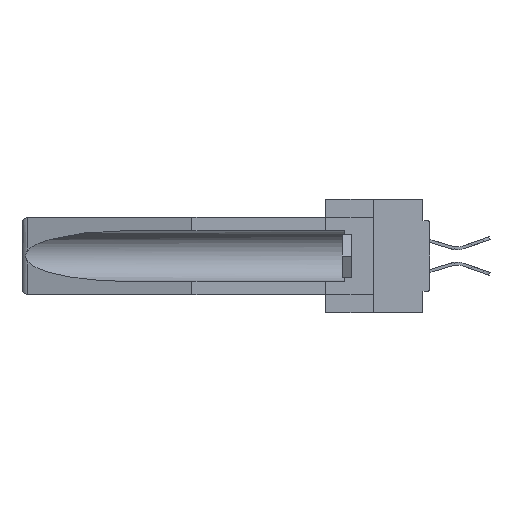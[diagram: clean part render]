
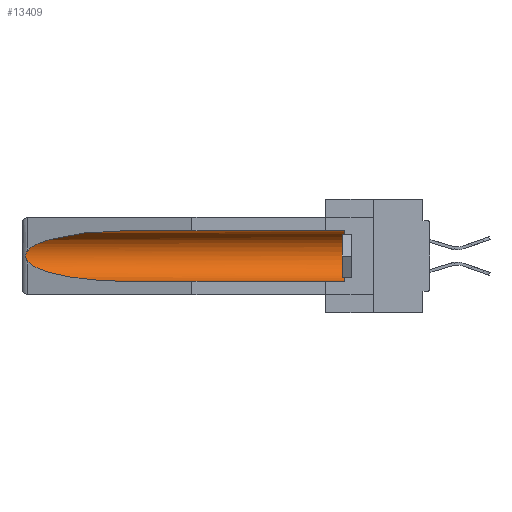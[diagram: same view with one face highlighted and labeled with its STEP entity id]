
A CAD part, left-side view. The second image highlights one B-rep face of the part: STEP entity #13409.
In plain terms, the highlighted cylindrical face has radius 2.857 mm (diameter 5.715 mm), a partial arc.
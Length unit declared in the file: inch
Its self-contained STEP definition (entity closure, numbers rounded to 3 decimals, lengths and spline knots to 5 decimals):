
#12 = AXIS2_PLACEMENT_3D ( 'NONE', #11659, #34735, #1858 ) ;
#1206 = CARTESIAN_POINT ( 'NONE',  ( 0.2675, 1.53308, -0.16763 ) ) ;
#1270 = DIRECTION ( 'NONE',  ( 0., 1., 0. ) ) ;
#1858 = DIRECTION ( 'NONE',  ( 0., 0., 1. ) ) ;
#2294 = CYLINDRICAL_SURFACE ( 'NONE', #33817, 0.1125 ) ;
#2442 = EDGE_CURVE ( 'NONE', #13617, #41362, #18137, .T. ) ;
#2776 = FACE_OUTER_BOUND ( 'NONE', #39328, .T. ) ;
#3018 = DIRECTION ( 'NONE',  ( 0., 1., 0. ) ) ;
#3958 = ORIENTED_EDGE ( 'NONE', *, *, #25917, .F. ) ;
#4309 = VECTOR ( 'NONE', #3018, 39.37008 ) ;
#4374 = CARTESIAN_POINT ( 'NONE',  ( 0.26654, 1.53092, -0.15636 ) ) ;
#5000 = CARTESIAN_POINT ( 'NONE',  ( 0.155, 1.07973, -0.284 ) ) ;
#5663 = CARTESIAN_POINT ( 'NONE',  ( 0.155, 0.126, -0.059 ) ) ;
#7551 = DIRECTION ( 'NONE',  ( 0., 0., 1. ) ) ;
#8029 = CARTESIAN_POINT ( 'NONE',  ( 0.21114, 1.30732, -0.284 ) ) ;
#8088 = EDGE_CURVE ( 'NONE', #12932, #9322, #22255, .T. ) ;
#8124 = EDGE_CURVE ( 'NONE', #18092, #32722, #23951, .T. ) ;
#9322 = VERTEX_POINT ( 'NONE', #5663 ) ;
#9747 = CARTESIAN_POINT ( 'NONE',  ( 0.155, -0.30754, -0.059 ) ) ;
#10079 = ORIENTED_EDGE ( 'NONE', *, *, #8088, .T. ) ;
#11659 = CARTESIAN_POINT ( 'NONE',  ( 0.155, 0.126, -0.1715 ) ) ;
#12932 = VERTEX_POINT ( 'NONE', #41295 ) ;
#13409 = ADVANCED_FACE ( 'NONE', ( #2776 ), #2294, .F. ) ;
#13617 = VERTEX_POINT ( 'NONE', #39685 ) ;
#14537 = CARTESIAN_POINT ( 'NONE',  ( 0.26537, 1.52718, -0.19328 ) ) ;
#15004 = ORIENTED_EDGE ( 'NONE', *, *, #2442, .T. ) ;
#15429 = CARTESIAN_POINT ( 'NONE',  ( 0.155, 1.07973, -0.059 ) ) ;
#15571 = CARTESIAN_POINT ( 'NONE',  ( 0.26537, 1.52718, -0.14972 ) ) ;
#16607 = CARTESIAN_POINT ( 'NONE',  ( 0.26537, 1.52718, -0.19328 ) ) ;
#17182 = LINE ( 'NONE', #9747, #4309 ) ;
#17464 = CARTESIAN_POINT ( 'NONE',  ( 0.26655, 1.53094, -0.18657 ) ) ;
#17824 = EDGE_CURVE ( 'NONE', #9322, #13617, #17182, .T. ) ;
#18092 = VERTEX_POINT ( 'NONE', #16607 ) ;
#18137 =( BOUNDED_CURVE ( )  B_SPLINE_CURVE ( 3, ( #15429, #19016, #18460, #15571 ),
 .UNSPECIFIED., .F., .F. ) 
 B_SPLINE_CURVE_WITH_KNOTS ( ( 4, 4 ),
 ( 4.71239, 6.08839 ),
 .UNSPECIFIED. ) 
 CURVE ( )  GEOMETRIC_REPRESENTATION_ITEM ( )  RATIONAL_B_SPLINE_CURVE ( ( 1., 0.848, 0.848, 1. ) ) 
 REPRESENTATION_ITEM ( '' )  );
#18460 = CARTESIAN_POINT ( 'NONE',  ( 0.25451, 1.48313, -0.09465 ) ) ;
#19016 = CARTESIAN_POINT ( 'NONE',  ( 0.21114, 1.30732, -0.059 ) ) ;
#19751 = EDGE_CURVE ( 'NONE', #41362, #18092, #32897, .T. ) ;
#20636 = CARTESIAN_POINT ( 'NONE',  ( 0.2673, 1.53269, -0.17917 ) ) ;
#22255 = CIRCLE ( 'NONE', #12, 0.1125 ) ;
#23951 =( BOUNDED_CURVE ( )  B_SPLINE_CURVE ( 3, ( #14537, #24899, #8029, #31212 ),
 .UNSPECIFIED., .F., .F. ) 
 B_SPLINE_CURVE_WITH_KNOTS ( ( 4, 4 ),
 ( 0.1948, 1.5708 ),
 .UNSPECIFIED. ) 
 CURVE ( )  GEOMETRIC_REPRESENTATION_ITEM ( )  RATIONAL_B_SPLINE_CURVE ( ( 1., 0.848, 0.848, 1. ) ) 
 REPRESENTATION_ITEM ( '' )  );
#24899 = CARTESIAN_POINT ( 'NONE',  ( 0.25451, 1.48313, -0.24835 ) ) ;
#24902 = LINE ( 'NONE', #37745, #33660 ) ;
#25917 = EDGE_CURVE ( 'NONE', #12932, #32722, #24902, .T. ) ;
#27378 = ORIENTED_EDGE ( 'NONE', *, *, #19751, .T. ) ;
#27522 = CARTESIAN_POINT ( 'NONE',  ( 0.26597, 1.5296, -0.19026 ) ) ;
#28574 = CARTESIAN_POINT ( 'NONE',  ( 0.26537, 1.52718, -0.14972 ) ) ;
#29623 = ORIENTED_EDGE ( 'NONE', *, *, #8124, .T. ) ;
#31212 = CARTESIAN_POINT ( 'NONE',  ( 0.155, 1.07973, -0.284 ) ) ;
#32722 = VERTEX_POINT ( 'NONE', #5000 ) ;
#32897 = B_SPLINE_CURVE_WITH_KNOTS ( 'NONE', 3,
 ( #34201, #37553, #4374, #33737, #1206, #37686, #20636, #17464, #27522, #41054 ),
 .UNSPECIFIED., .F., .F.,
 ( 4, 2, 2, 2, 4 ),
 ( 0., 0.00029, 0.00058, 0.00087, 0.00117 ),
 .UNSPECIFIED. ) ;
#33660 = VECTOR ( 'NONE', #1270, 39.37008 ) ;
#33737 = CARTESIAN_POINT ( 'NONE',  ( 0.2673, 1.5327, -0.16383 ) ) ;
#33817 = AXIS2_PLACEMENT_3D ( 'NONE', #40376, #40522, #7551 ) ;
#34201 = CARTESIAN_POINT ( 'NONE',  ( 0.26537, 1.52718, -0.14972 ) ) ;
#34631 = ORIENTED_EDGE ( 'NONE', *, *, #17824, .T. ) ;
#34735 = DIRECTION ( 'NONE',  ( 0., -1., 0. ) ) ;
#37553 = CARTESIAN_POINT ( 'NONE',  ( 0.26597, 1.52961, -0.15275 ) ) ;
#37686 = CARTESIAN_POINT ( 'NONE',  ( 0.2675, 1.53308, -0.17534 ) ) ;
#37745 = CARTESIAN_POINT ( 'NONE',  ( 0.155, -0.30754, -0.284 ) ) ;
#39328 = EDGE_LOOP ( 'NONE', ( #15004, #27378, #29623, #3958, #10079, #34631 ) ) ;
#39685 = CARTESIAN_POINT ( 'NONE',  ( 0.155, 1.07973, -0.059 ) ) ;
#40376 = CARTESIAN_POINT ( 'NONE',  ( 0.155, -0.30754, -0.1715 ) ) ;
#40522 = DIRECTION ( 'NONE',  ( 0., 1., 0. ) ) ;
#41054 = CARTESIAN_POINT ( 'NONE',  ( 0.26537, 1.52718, -0.19328 ) ) ;
#41295 = CARTESIAN_POINT ( 'NONE',  ( 0.155, 0.126, -0.284 ) ) ;
#41362 = VERTEX_POINT ( 'NONE', #28574 ) ;
